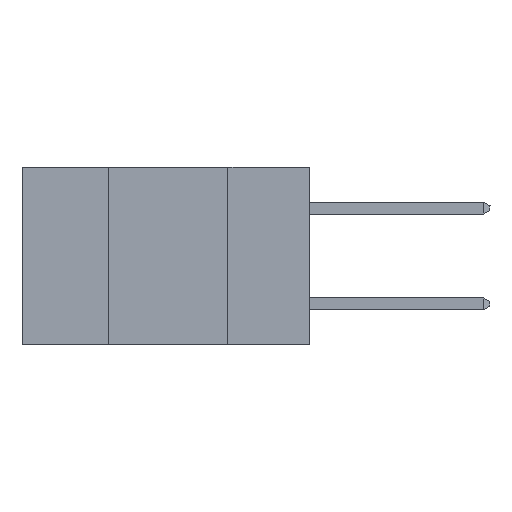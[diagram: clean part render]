
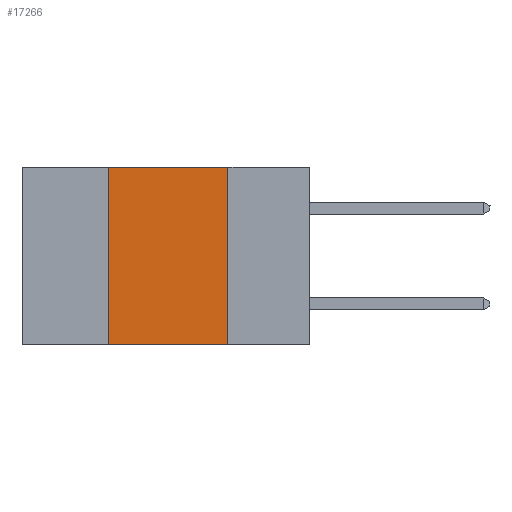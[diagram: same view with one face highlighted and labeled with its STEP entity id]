
A CAD part, left-side view. The second image highlights one B-rep face of the part: STEP entity #17266.
In plain terms, the highlighted planar face has unit normal (-1, 0, 0).
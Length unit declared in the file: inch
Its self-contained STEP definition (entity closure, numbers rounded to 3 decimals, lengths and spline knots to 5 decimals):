
#154 = ORIENTED_EDGE ( 'NONE', *, *, #9486, .F. ) ;
#367 = DIRECTION ( 'NONE',  ( 0., 0., 1. ) ) ;
#512 = DIRECTION ( 'NONE',  ( 0., -1., 0. ) ) ;
#694 = LINE ( 'NONE', #18439, #12616 ) ;
#824 = LINE ( 'NONE', #14518, #2273 ) ;
#1139 = AXIS2_PLACEMENT_3D ( 'NONE', #18754, #17031, #10963 ) ;
#2198 = EDGE_CURVE ( 'NONE', #17131, #11873, #824, .T. ) ;
#2273 = VECTOR ( 'NONE', #367, 39.37008 ) ;
#2282 = ORIENTED_EDGE ( 'NONE', *, *, #17417, .F. ) ;
#2540 = ORIENTED_EDGE ( 'NONE', *, *, #8990, .T. ) ;
#3596 = FACE_OUTER_BOUND ( 'NONE', #19936, .T. ) ;
#4059 = LINE ( 'NONE', #11138, #6499 ) ;
#5893 = VERTEX_POINT ( 'NONE', #18268 ) ;
#6279 = PLANE ( 'NONE',  #1139 ) ;
#6499 = VECTOR ( 'NONE', #512, 39.37008 ) ;
#8990 = EDGE_CURVE ( 'NONE', #17131, #11626, #694, .T. ) ;
#9486 = EDGE_CURVE ( 'NONE', #11873, #5893, #4059, .T. ) ;
#10963 = DIRECTION ( 'NONE',  ( 0., 0., -1. ) ) ;
#11138 = CARTESIAN_POINT ( 'NONE',  ( 0., 0.6, 0. ) ) ;
#11626 = VERTEX_POINT ( 'NONE', #17045 ) ;
#11873 = VERTEX_POINT ( 'NONE', #15921 ) ;
#12616 = VECTOR ( 'NONE', #20000, 39.37008 ) ;
#13203 = DIRECTION ( 'NONE',  ( 0., 0., -1. ) ) ;
#14518 = CARTESIAN_POINT ( 'NONE',  ( 0., 0.42, 0. ) ) ;
#15543 = CARTESIAN_POINT ( 'NONE',  ( 0., 0.17, 0. ) ) ;
#15921 = CARTESIAN_POINT ( 'NONE',  ( 0., 0.42, 0. ) ) ;
#16192 = VECTOR ( 'NONE', #13203, 39.37008 ) ;
#17031 = DIRECTION ( 'NONE',  ( 1., 0., 0. ) ) ;
#17045 = CARTESIAN_POINT ( 'NONE',  ( 0., 0.17, -0.37 ) ) ;
#17046 = ORIENTED_EDGE ( 'NONE', *, *, #2198, .F. ) ;
#17131 = VERTEX_POINT ( 'NONE', #18421 ) ;
#17266 = ADVANCED_FACE ( 'NONE', ( #3596 ), #6279, .F. ) ;
#17417 = EDGE_CURVE ( 'NONE', #5893, #11626, #18837, .T. ) ;
#18268 = CARTESIAN_POINT ( 'NONE',  ( 0., 0.17, 0. ) ) ;
#18421 = CARTESIAN_POINT ( 'NONE',  ( 0., 0.42, -0.37 ) ) ;
#18439 = CARTESIAN_POINT ( 'NONE',  ( 0., 0.6, -0.37 ) ) ;
#18754 = CARTESIAN_POINT ( 'NONE',  ( 0., 0.6, 0. ) ) ;
#18837 = LINE ( 'NONE', #15543, #16192 ) ;
#19936 = EDGE_LOOP ( 'NONE', ( #2282, #154, #17046, #2540 ) ) ;
#20000 = DIRECTION ( 'NONE',  ( 0., -1., 0. ) ) ;
